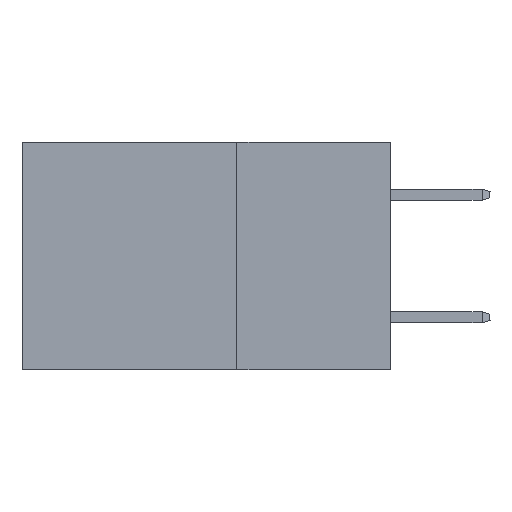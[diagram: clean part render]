
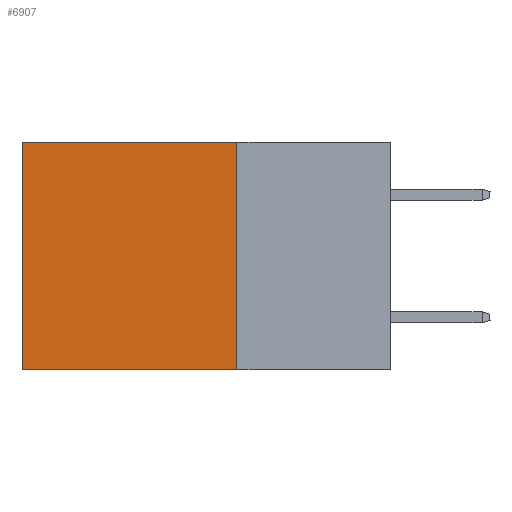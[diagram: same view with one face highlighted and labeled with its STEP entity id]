
A CAD part, left-side view. The second image highlights one B-rep face of the part: STEP entity #6907.
In plain terms, the highlighted planar face has unit normal (-1, 0, 0).
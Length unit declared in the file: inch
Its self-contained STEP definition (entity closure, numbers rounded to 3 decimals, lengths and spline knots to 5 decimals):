
#53 = CARTESIAN_POINT ( 'NONE',  ( 0.2875, 0.6, 0. ) ) ;
#68 = DIRECTION ( 'NONE',  ( 0., 0., -1. ) ) ;
#420 = VECTOR ( 'NONE', #7593, 39.37008 ) ;
#613 = CARTESIAN_POINT ( 'NONE',  ( 0.2875, 0.25, 0. ) ) ;
#760 = DIRECTION ( 'NONE',  ( 0., 1., 0. ) ) ;
#802 = VERTEX_POINT ( 'NONE', #4919 ) ;
#1111 = EDGE_CURVE ( 'NONE', #3544, #4074, #8568, .T. ) ;
#1487 = VERTEX_POINT ( 'NONE', #7947 ) ;
#2109 = VECTOR ( 'NONE', #6543, 39.37008 ) ;
#2498 = PLANE ( 'NONE',  #7059 ) ;
#2878 = DIRECTION ( 'NONE',  ( 0., 0., -1. ) ) ;
#3409 = DIRECTION ( 'NONE',  ( 1., 0., 0. ) ) ;
#3438 = CARTESIAN_POINT ( 'NONE',  ( 0.2875, 0.25, 0. ) ) ;
#3544 = VERTEX_POINT ( 'NONE', #8517 ) ;
#3570 = CARTESIAN_POINT ( 'NONE',  ( 0.2875, 0.6, -0.37 ) ) ;
#4074 = VERTEX_POINT ( 'NONE', #3570 ) ;
#4433 = EDGE_CURVE ( 'NONE', #802, #3544, #6542, .T. ) ;
#4919 = CARTESIAN_POINT ( 'NONE',  ( 0.2875, 0.25, 0. ) ) ;
#5368 = FACE_OUTER_BOUND ( 'NONE', #7892, .T. ) ;
#5833 = CARTESIAN_POINT ( 'NONE',  ( 0.2875, 0.25, 0. ) ) ;
#6079 = EDGE_CURVE ( 'NONE', #802, #1487, #8041, .T. ) ;
#6542 = LINE ( 'NONE', #613, #8390 ) ;
#6543 = DIRECTION ( 'NONE',  ( 0., 0., -1. ) ) ;
#6907 = ADVANCED_FACE ( 'NONE', ( #5368 ), #2498, .F. ) ;
#7059 = AXIS2_PLACEMENT_3D ( 'NONE', #3438, #3409, #2878 ) ;
#7387 = ORIENTED_EDGE ( 'NONE', *, *, #1111, .T. ) ;
#7428 = ORIENTED_EDGE ( 'NONE', *, *, #9547, .F. ) ;
#7435 = ORIENTED_EDGE ( 'NONE', *, *, #6079, .F. ) ;
#7444 = ORIENTED_EDGE ( 'NONE', *, *, #4433, .T. ) ;
#7593 = DIRECTION ( 'NONE',  ( 0., 1., 0. ) ) ;
#7892 = EDGE_LOOP ( 'NONE', ( #7387, #7428, #7435, #7444 ) ) ;
#7947 = CARTESIAN_POINT ( 'NONE',  ( 0.2875, 0.25, -0.37 ) ) ;
#8041 = LINE ( 'NONE', #5833, #2109 ) ;
#8199 = LINE ( 'NONE', #8958, #420 ) ;
#8390 = VECTOR ( 'NONE', #760, 39.37008 ) ;
#8517 = CARTESIAN_POINT ( 'NONE',  ( 0.2875, 0.6, 0. ) ) ;
#8568 = LINE ( 'NONE', #53, #8763 ) ;
#8763 = VECTOR ( 'NONE', #68, 39.37008 ) ;
#8958 = CARTESIAN_POINT ( 'NONE',  ( 0.2875, 0.25, -0.37 ) ) ;
#9547 = EDGE_CURVE ( 'NONE', #1487, #4074, #8199, .T. ) ;
